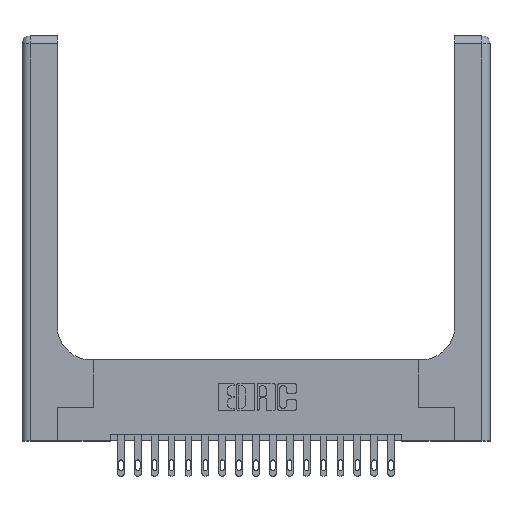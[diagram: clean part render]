
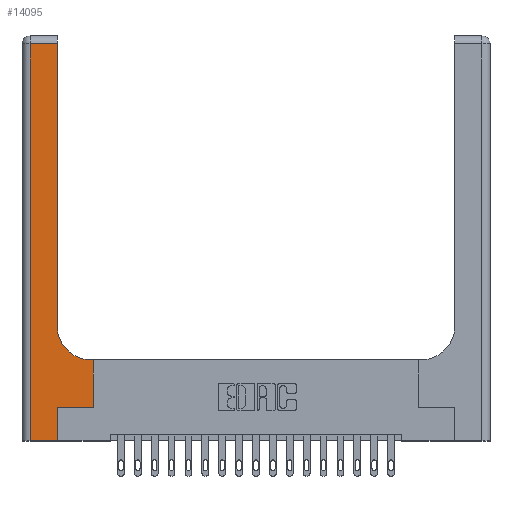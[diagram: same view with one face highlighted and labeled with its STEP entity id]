
A CAD part, top view. The second image highlights one B-rep face of the part: STEP entity #14095.
In plain terms, the highlighted planar face has unit normal (0, 0, 1).
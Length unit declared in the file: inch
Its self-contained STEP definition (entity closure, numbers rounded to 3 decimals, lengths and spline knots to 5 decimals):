
#367 = CARTESIAN_POINT ( 'NONE',  ( 0.06, 2.94, 0.37 ) ) ;
#444 = LINE ( 'NONE', #14330, #17762 ) ;
#497 = LINE ( 'NONE', #11164, #12850 ) ;
#873 = VECTOR ( 'NONE', #16715, 39.37008 ) ;
#1265 = VECTOR ( 'NONE', #6746, 39.37008 ) ;
#1357 = ORIENTED_EDGE ( 'NONE', *, *, #10344, .T. ) ;
#1479 = VERTEX_POINT ( 'NONE', #9552 ) ;
#2100 = CARTESIAN_POINT ( 'NONE',  ( 0.528, 0.25, 0.37 ) ) ;
#2865 = VERTEX_POINT ( 'NONE', #19742 ) ;
#3863 = CARTESIAN_POINT ( 'NONE',  ( 0.06, 0., 0.37 ) ) ;
#4053 = VECTOR ( 'NONE', #11035, 39.37008 ) ;
#4109 = CIRCLE ( 'NONE', #18345, 0.25 ) ;
#4208 = EDGE_CURVE ( 'NONE', #2865, #4308, #6179, .T. ) ;
#4298 = EDGE_CURVE ( 'NONE', #9563, #9255, #9998, .T. ) ;
#4308 = VERTEX_POINT ( 'NONE', #367 ) ;
#5389 = ORIENTED_EDGE ( 'NONE', *, *, #8677, .T. ) ;
#5500 = CARTESIAN_POINT ( 'NONE',  ( 0.51, 0.6, 0.37 ) ) ;
#5614 = CARTESIAN_POINT ( 'NONE',  ( 0.528, 0.6, 0.37 ) ) ;
#6026 = ORIENTED_EDGE ( 'NONE', *, *, #14639, .T. ) ;
#6179 = LINE ( 'NONE', #7790, #4053 ) ;
#6383 = ORIENTED_EDGE ( 'NONE', *, *, #4298, .T. ) ;
#6471 = PLANE ( 'NONE',  #16230 ) ;
#6503 = LINE ( 'NONE', #19056, #13850 ) ;
#6704 = DIRECTION ( 'NONE',  ( 0., 1., 0. ) ) ;
#6714 = DIRECTION ( 'NONE',  ( 1., 0., 0. ) ) ;
#6746 = DIRECTION ( 'NONE',  ( -1., 0., 0. ) ) ;
#6808 = VERTEX_POINT ( 'NONE', #13895 ) ;
#6832 = DIRECTION ( 'NONE',  ( 0., 0., -1. ) ) ;
#6956 = EDGE_CURVE ( 'NONE', #9255, #1479, #497, .T. ) ;
#7790 = CARTESIAN_POINT ( 'NONE',  ( 0., 2.94, 0.37 ) ) ;
#7801 = EDGE_CURVE ( 'NONE', #18102, #6808, #4109, .T. ) ;
#8086 = DIRECTION ( 'NONE',  ( 0., 0., -1. ) ) ;
#8096 = VECTOR ( 'NONE', #15829, 39.37008 ) ;
#8565 = LINE ( 'NONE', #14744, #1265 ) ;
#8677 = EDGE_CURVE ( 'NONE', #4308, #9563, #17019, .T. ) ;
#9255 = VERTEX_POINT ( 'NONE', #19000 ) ;
#9552 = CARTESIAN_POINT ( 'NONE',  ( 0.265, 0.25, 0.37 ) ) ;
#9555 = EDGE_CURVE ( 'NONE', #1479, #10024, #6503, .T. ) ;
#9563 = VERTEX_POINT ( 'NONE', #3863 ) ;
#9698 = FACE_OUTER_BOUND ( 'NONE', #14933, .T. ) ;
#9861 = VECTOR ( 'NONE', #16177, 39.37008 ) ;
#9998 = LINE ( 'NONE', #17501, #9861 ) ;
#10024 = VERTEX_POINT ( 'NONE', #2100 ) ;
#10344 = EDGE_CURVE ( 'NONE', #6808, #2865, #444, .T. ) ;
#10485 = EDGE_CURVE ( 'NONE', #14829, #18102, #8565, .T. ) ;
#10552 = CARTESIAN_POINT ( 'NONE',  ( 0.06, 3., 0.37 ) ) ;
#11035 = DIRECTION ( 'NONE',  ( -1., 0., 0. ) ) ;
#11164 = CARTESIAN_POINT ( 'NONE',  ( 0.265, 0., 0.37 ) ) ;
#12692 = CARTESIAN_POINT ( 'NONE',  ( 0.51, 0.85, 0.37 ) ) ;
#12850 = VECTOR ( 'NONE', #6704, 39.37008 ) ;
#13104 = ORIENTED_EDGE ( 'NONE', *, *, #9555, .T. ) ;
#13850 = VECTOR ( 'NONE', #6714, 39.37008 ) ;
#13895 = CARTESIAN_POINT ( 'NONE',  ( 0.26, 0.85, 0.37 ) ) ;
#14012 = ORIENTED_EDGE ( 'NONE', *, *, #4208, .T. ) ;
#14095 = ADVANCED_FACE ( 'NONE', ( #9698 ), #6471, .F. ) ;
#14131 = ORIENTED_EDGE ( 'NONE', *, *, #10485, .T. ) ;
#14330 = CARTESIAN_POINT ( 'NONE',  ( 0.26, 3., 0.37 ) ) ;
#14454 = ORIENTED_EDGE ( 'NONE', *, *, #6956, .T. ) ;
#14638 = LINE ( 'NONE', #17567, #8096 ) ;
#14639 = EDGE_CURVE ( 'NONE', #10024, #14829, #14638, .T. ) ;
#14744 = CARTESIAN_POINT ( 'NONE',  ( 0.26, 0.6, 0.37 ) ) ;
#14829 = VERTEX_POINT ( 'NONE', #5614 ) ;
#14933 = EDGE_LOOP ( 'NONE', ( #1357, #14012, #5389, #6383, #14454, #13104, #6026, #14131, #15196 ) ) ;
#15196 = ORIENTED_EDGE ( 'NONE', *, *, #7801, .T. ) ;
#15774 = CARTESIAN_POINT ( 'NONE',  ( 0., 3., 0.37 ) ) ;
#15829 = DIRECTION ( 'NONE',  ( 0., 1., 0. ) ) ;
#16177 = DIRECTION ( 'NONE',  ( 1., 0., 0. ) ) ;
#16230 = AXIS2_PLACEMENT_3D ( 'NONE', #15774, #8086, #18726 ) ;
#16715 = DIRECTION ( 'NONE',  ( 0., -1., 0. ) ) ;
#17019 = LINE ( 'NONE', #10552, #873 ) ;
#17482 = DIRECTION ( 'NONE',  ( 0., 1., 0. ) ) ;
#17501 = CARTESIAN_POINT ( 'NONE',  ( 0., 0., 0.37 ) ) ;
#17567 = CARTESIAN_POINT ( 'NONE',  ( 0.528, 0.25, 0.37 ) ) ;
#17762 = VECTOR ( 'NONE', #17482, 39.37008 ) ;
#18102 = VERTEX_POINT ( 'NONE', #5500 ) ;
#18345 = AXIS2_PLACEMENT_3D ( 'NONE', #12692, #6832, #19278 ) ;
#18726 = DIRECTION ( 'NONE',  ( -1., 0., 0. ) ) ;
#19000 = CARTESIAN_POINT ( 'NONE',  ( 0.265, 0., 0.37 ) ) ;
#19056 = CARTESIAN_POINT ( 'NONE',  ( 0.265, 0.25, 0.37 ) ) ;
#19278 = DIRECTION ( 'NONE',  ( 1., 0., 0. ) ) ;
#19742 = CARTESIAN_POINT ( 'NONE',  ( 0.26, 2.94, 0.37 ) ) ;
